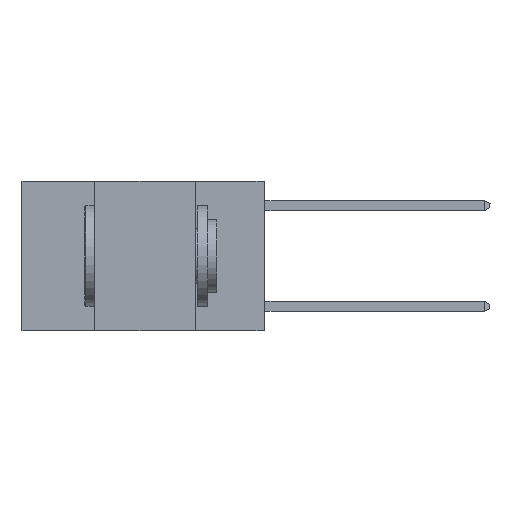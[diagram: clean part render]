
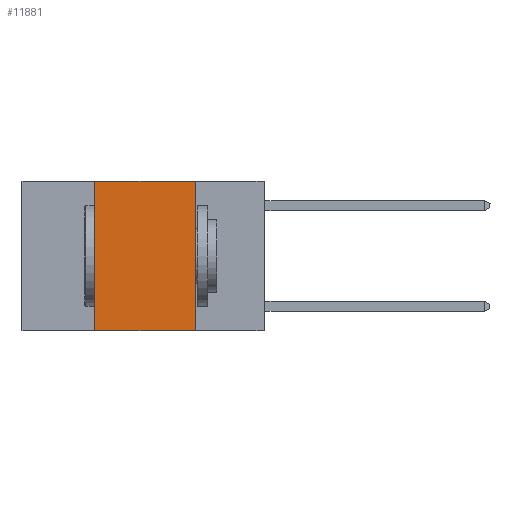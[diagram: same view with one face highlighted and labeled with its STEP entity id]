
A CAD part, left-side view. The second image highlights one B-rep face of the part: STEP entity #11881.
In plain terms, the highlighted planar face has unit normal (-1, 0, 0).
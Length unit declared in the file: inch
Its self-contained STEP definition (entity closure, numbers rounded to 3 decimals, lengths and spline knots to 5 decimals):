
#67 = PLANE ( 'NONE',  #2673 ) ;
#987 = VERTEX_POINT ( 'NONE', #13971 ) ;
#1279 = VERTEX_POINT ( 'NONE', #5758 ) ;
#1300 = DIRECTION ( 'NONE',  ( 1., 0., 0. ) ) ;
#1449 = DIRECTION ( 'NONE',  ( 0., 0., -1. ) ) ;
#2296 = LINE ( 'NONE', #6455, #9591 ) ;
#2316 = CARTESIAN_POINT ( 'NONE',  ( 0., 0.6, 0. ) ) ;
#2673 = AXIS2_PLACEMENT_3D ( 'NONE', #2316, #1300, #1449 ) ;
#2883 = LINE ( 'NONE', #4103, #7238 ) ;
#3060 = VERTEX_POINT ( 'NONE', #5395 ) ;
#3272 = ORIENTED_EDGE ( 'NONE', *, *, #10629, .F. ) ;
#4103 = CARTESIAN_POINT ( 'NONE',  ( 0., 0.6, 0. ) ) ;
#4308 = FACE_OUTER_BOUND ( 'NONE', #8896, .T. ) ;
#4332 = VECTOR ( 'NONE', #5512, 39.37008 ) ;
#5395 = CARTESIAN_POINT ( 'NONE',  ( 0., 0.42, 0. ) ) ;
#5495 = EDGE_CURVE ( 'NONE', #3060, #987, #2883, .T. ) ;
#5512 = DIRECTION ( 'NONE',  ( 0., 0., 1. ) ) ;
#5673 = ORIENTED_EDGE ( 'NONE', *, *, #7934, .F. ) ;
#5758 = CARTESIAN_POINT ( 'NONE',  ( 0., 0.42, -0.37 ) ) ;
#6455 = CARTESIAN_POINT ( 'NONE',  ( 0., 0.17, 0. ) ) ;
#6467 = EDGE_CURVE ( 'NONE', #1279, #13955, #13497, .T. ) ;
#7033 = CARTESIAN_POINT ( 'NONE',  ( 0., 0.6, -0.37 ) ) ;
#7238 = VECTOR ( 'NONE', #7260, 39.37008 ) ;
#7260 = DIRECTION ( 'NONE',  ( 0., -1., 0. ) ) ;
#7328 = ORIENTED_EDGE ( 'NONE', *, *, #6467, .T. ) ;
#7362 = CARTESIAN_POINT ( 'NONE',  ( 0., 0.17, -0.37 ) ) ;
#7934 = EDGE_CURVE ( 'NONE', #987, #13955, #2296, .T. ) ;
#8280 = ORIENTED_EDGE ( 'NONE', *, *, #5495, .F. ) ;
#8896 = EDGE_LOOP ( 'NONE', ( #5673, #8280, #3272, #7328 ) ) ;
#9318 = DIRECTION ( 'NONE',  ( 0., 0., -1. ) ) ;
#9591 = VECTOR ( 'NONE', #9318, 39.37008 ) ;
#9972 = LINE ( 'NONE', #13204, #4332 ) ;
#10629 = EDGE_CURVE ( 'NONE', #1279, #3060, #9972, .T. ) ;
#11881 = ADVANCED_FACE ( 'NONE', ( #4308 ), #67, .F. ) ;
#12090 = VECTOR ( 'NONE', #12454, 39.37008 ) ;
#12454 = DIRECTION ( 'NONE',  ( 0., -1., 0. ) ) ;
#13204 = CARTESIAN_POINT ( 'NONE',  ( 0., 0.42, 0. ) ) ;
#13497 = LINE ( 'NONE', #7033, #12090 ) ;
#13955 = VERTEX_POINT ( 'NONE', #7362 ) ;
#13971 = CARTESIAN_POINT ( 'NONE',  ( 0., 0.17, 0. ) ) ;
